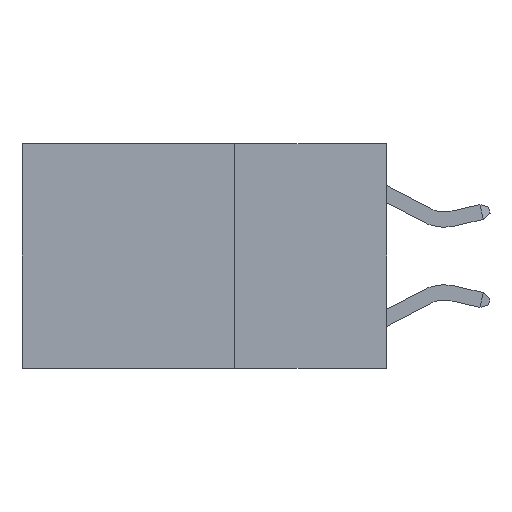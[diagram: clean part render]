
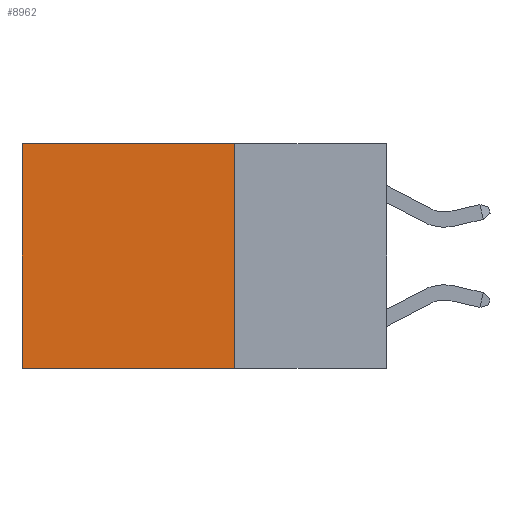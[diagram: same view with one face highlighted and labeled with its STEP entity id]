
A CAD part, left-side view. The second image highlights one B-rep face of the part: STEP entity #8962.
In plain terms, the highlighted planar face has unit normal (-1, 0, 0).
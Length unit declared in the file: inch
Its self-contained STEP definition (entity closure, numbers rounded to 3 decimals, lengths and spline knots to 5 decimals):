
#19 = DIRECTION ( 'NONE',  ( 0., 0., -1. ) ) ;
#535 = EDGE_CURVE ( 'NONE', #8741, #11049, #4898, .T. ) ;
#663 = VECTOR ( 'NONE', #3046, 39.37008 ) ;
#1021 = VECTOR ( 'NONE', #19, 39.37008 ) ;
#1123 = ORIENTED_EDGE ( 'NONE', *, *, #13472, .F. ) ;
#1359 = CARTESIAN_POINT ( 'NONE',  ( 0.2625, 0.25, 0. ) ) ;
#1511 = CARTESIAN_POINT ( 'NONE',  ( 0.2625, 0.25, -0.37 ) ) ;
#2023 = CARTESIAN_POINT ( 'NONE',  ( 0.2625, 0.6, 0. ) ) ;
#2766 = ORIENTED_EDGE ( 'NONE', *, *, #6019, .T. ) ;
#2817 = DIRECTION ( 'NONE',  ( 1., 0., 0. ) ) ;
#3046 = DIRECTION ( 'NONE',  ( 0., 1., 0. ) ) ;
#4415 = CARTESIAN_POINT ( 'NONE',  ( 0.2625, 0.25, 0. ) ) ;
#4898 = LINE ( 'NONE', #5718, #1021 ) ;
#5718 = CARTESIAN_POINT ( 'NONE',  ( 0.2625, 0.25, 0. ) ) ;
#5814 = ORIENTED_EDGE ( 'NONE', *, *, #535, .F. ) ;
#6019 = EDGE_CURVE ( 'NONE', #8741, #10898, #8985, .T. ) ;
#7045 = CARTESIAN_POINT ( 'NONE',  ( 0.2625, 0.25, -0.37 ) ) ;
#7263 = AXIS2_PLACEMENT_3D ( 'NONE', #1359, #2817, #14655 ) ;
#7523 = CARTESIAN_POINT ( 'NONE',  ( 0.2625, 0.6, -0.37 ) ) ;
#8741 = VERTEX_POINT ( 'NONE', #4415 ) ;
#8898 = EDGE_LOOP ( 'NONE', ( #14630, #1123, #5814, #2766 ) ) ;
#8962 = ADVANCED_FACE ( 'NONE', ( #14144 ), #10300, .F. ) ;
#8985 = LINE ( 'NONE', #17310, #11045 ) ;
#9034 = LINE ( 'NONE', #1511, #663 ) ;
#10237 = VECTOR ( 'NONE', #14876, 39.37008 ) ;
#10300 = PLANE ( 'NONE',  #7263 ) ;
#10898 = VERTEX_POINT ( 'NONE', #12543 ) ;
#11045 = VECTOR ( 'NONE', #13022, 39.37008 ) ;
#11049 = VERTEX_POINT ( 'NONE', #7045 ) ;
#12543 = CARTESIAN_POINT ( 'NONE',  ( 0.2625, 0.6, 0. ) ) ;
#13022 = DIRECTION ( 'NONE',  ( 0., 1., 0. ) ) ;
#13472 = EDGE_CURVE ( 'NONE', #11049, #18674, #9034, .T. ) ;
#14144 = FACE_OUTER_BOUND ( 'NONE', #8898, .T. ) ;
#14630 = ORIENTED_EDGE ( 'NONE', *, *, #17357, .T. ) ;
#14655 = DIRECTION ( 'NONE',  ( 0., 0., -1. ) ) ;
#14876 = DIRECTION ( 'NONE',  ( 0., 0., -1. ) ) ;
#17310 = CARTESIAN_POINT ( 'NONE',  ( 0.2625, 0.25, 0. ) ) ;
#17357 = EDGE_CURVE ( 'NONE', #10898, #18674, #18486, .T. ) ;
#18486 = LINE ( 'NONE', #2023, #10237 ) ;
#18674 = VERTEX_POINT ( 'NONE', #7523 ) ;
